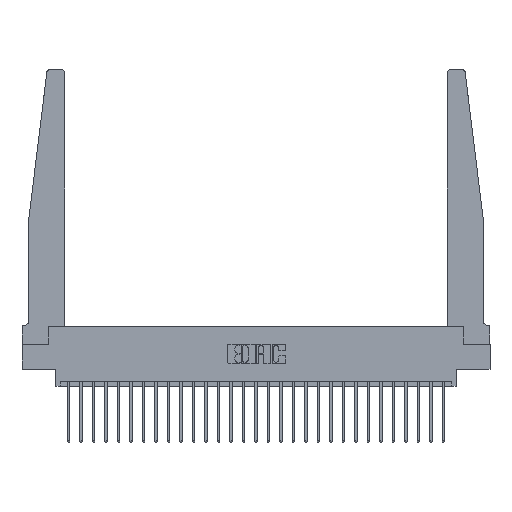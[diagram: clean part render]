
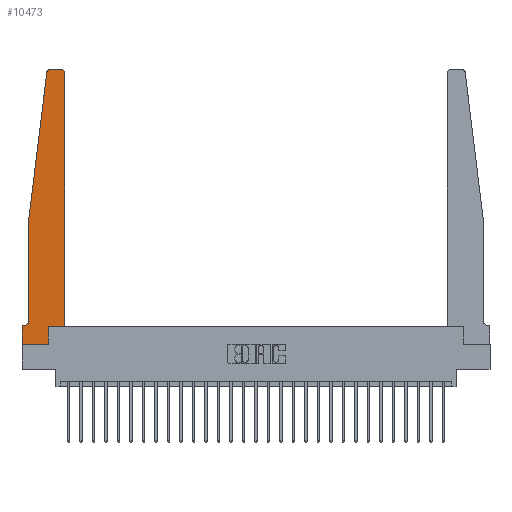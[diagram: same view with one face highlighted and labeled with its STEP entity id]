
A CAD part, top view. The second image highlights one B-rep face of the part: STEP entity #10473.
In plain terms, the highlighted planar face has unit normal (0, 0, 1).
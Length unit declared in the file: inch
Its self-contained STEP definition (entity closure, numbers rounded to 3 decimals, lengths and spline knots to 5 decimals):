
#105 = LINE ( 'NONE', #6262, #20757 ) ;
#352 = VERTEX_POINT ( 'NONE', #3799 ) ;
#757 = CARTESIAN_POINT ( 'NONE',  ( 0.065, 1.25, 0.37 ) ) ;
#1138 = CARTESIAN_POINT ( 'NONE',  ( 0.395, 2.72, 0.37 ) ) ;
#1237 = DIRECTION ( 'NONE',  ( 1., 0., 0. ) ) ;
#1488 = ORIENTED_EDGE ( 'NONE', *, *, #17526, .T. ) ;
#1494 = ORIENTED_EDGE ( 'NONE', *, *, #16974, .T. ) ;
#1615 = CARTESIAN_POINT ( 'NONE',  ( 0.425, 0.18, 0.37 ) ) ;
#2201 = VECTOR ( 'NONE', #18265, 39.37008 ) ;
#2873 = LINE ( 'NONE', #10935, #26638 ) ;
#2919 = ORIENTED_EDGE ( 'NONE', *, *, #4699, .T. ) ;
#3592 = DIRECTION ( 'NONE',  ( 0., 0., 1. ) ) ;
#3613 = CIRCLE ( 'NONE', #23729, 0.03 ) ;
#3799 = CARTESIAN_POINT ( 'NONE',  ( 0.27653, 2.75, 0.37 ) ) ;
#4699 = EDGE_CURVE ( 'NONE', #25485, #17885, #25501, .T. ) ;
#5096 = LINE ( 'NONE', #9466, #15453 ) ;
#5494 = EDGE_CURVE ( 'NONE', #25821, #16627, #105, .T. ) ;
#6005 = VERTEX_POINT ( 'NONE', #8654 ) ;
#6227 = EDGE_CURVE ( 'NONE', #9576, #12575, #3613, .T. ) ;
#6262 = CARTESIAN_POINT ( 'NONE',  ( 0.065, 1.25, 0.37 ) ) ;
#6812 = ORIENTED_EDGE ( 'NONE', *, *, #6227, .T. ) ;
#7024 = VECTOR ( 'NONE', #26680, 39.37008 ) ;
#7079 = EDGE_CURVE ( 'NONE', #22686, #25821, #5096, .T. ) ;
#7108 = CARTESIAN_POINT ( 'NONE',  ( 0., 0., 0.37 ) ) ;
#7135 = CARTESIAN_POINT ( 'NONE',  ( 0.425, 0.18, 0.37 ) ) ;
#7445 = DIRECTION ( 'NONE',  ( -1., 0., 0. ) ) ;
#7913 = DIRECTION ( 'NONE',  ( 0., -1., 0. ) ) ;
#8013 = CARTESIAN_POINT ( 'NONE',  ( 0.2605, 0., 0.37 ) ) ;
#8654 = CARTESIAN_POINT ( 'NONE',  ( 0., 0., 0.37 ) ) ;
#8744 = CARTESIAN_POINT ( 'NONE',  ( 0.24675, 2.72367, 0.37 ) ) ;
#9374 = ORIENTED_EDGE ( 'NONE', *, *, #5494, .T. ) ;
#9390 = CIRCLE ( 'NONE', #17277, 0.05 ) ;
#9466 = CARTESIAN_POINT ( 'NONE',  ( 0.065, 1.25, 0.37 ) ) ;
#9576 = VERTEX_POINT ( 'NONE', #15821 ) ;
#9884 = CARTESIAN_POINT ( 'NONE',  ( 0., 0., 0.37 ) ) ;
#10202 = VERTEX_POINT ( 'NONE', #23165 ) ;
#10473 = ADVANCED_FACE ( 'NONE', ( #23562 ), #24241, .T. ) ;
#10711 = EDGE_CURVE ( 'NONE', #6005, #17638, #11946, .T. ) ;
#10935 = CARTESIAN_POINT ( 'NONE',  ( 0.2605, 0.18, 0.37 ) ) ;
#11298 = ORIENTED_EDGE ( 'NONE', *, *, #25918, .T. ) ;
#11534 = DIRECTION ( 'NONE',  ( 1., 0., 0. ) ) ;
#11568 = LINE ( 'NONE', #11698, #14155 ) ;
#11698 = CARTESIAN_POINT ( 'NONE',  ( 0.065, 0.1875, 0.37 ) ) ;
#11766 = AXIS2_PLACEMENT_3D ( 'NONE', #22343, #18239, #20282 ) ;
#11946 = LINE ( 'NONE', #9884, #2201 ) ;
#12575 = VERTEX_POINT ( 'NONE', #14511 ) ;
#12731 = CARTESIAN_POINT ( 'NONE',  ( 0.2605, 0.18, 0.37 ) ) ;
#13665 = CARTESIAN_POINT ( 'NONE',  ( 0.015, 0.1875, 0.37 ) ) ;
#13770 = VECTOR ( 'NONE', #25782, 39.37008 ) ;
#13800 = EDGE_CURVE ( 'NONE', #16627, #20549, #9390, .T. ) ;
#14101 = VECTOR ( 'NONE', #23703, 39.37008 ) ;
#14127 = CARTESIAN_POINT ( 'NONE',  ( 0.425, 0.18, 0.37 ) ) ;
#14155 = VECTOR ( 'NONE', #7445, 39.37008 ) ;
#14511 = CARTESIAN_POINT ( 'NONE',  ( 0.395, 2.75, 0.37 ) ) ;
#15185 = ORIENTED_EDGE ( 'NONE', *, *, #23806, .T. ) ;
#15453 = VECTOR ( 'NONE', #15777, 39.37008 ) ;
#15749 = CARTESIAN_POINT ( 'NONE',  ( 0., 0.1875, 0.37 ) ) ;
#15777 = DIRECTION ( 'NONE',  ( -0.122, -0.992, 0. ) ) ;
#15821 = CARTESIAN_POINT ( 'NONE',  ( 0.425, 2.72, 0.37 ) ) ;
#16141 = ORIENTED_EDGE ( 'NONE', *, *, #23557, .T. ) ;
#16627 = VERTEX_POINT ( 'NONE', #21417 ) ;
#16889 = ORIENTED_EDGE ( 'NONE', *, *, #10711, .T. ) ;
#16974 = EDGE_CURVE ( 'NONE', #10202, #6005, #25893, .T. ) ;
#17246 = DIRECTION ( 'NONE',  ( 0., 1., 0. ) ) ;
#17277 = AXIS2_PLACEMENT_3D ( 'NONE', #21159, #25810, #19240 ) ;
#17526 = EDGE_CURVE ( 'NONE', #17885, #9576, #22290, .T. ) ;
#17602 = ORIENTED_EDGE ( 'NONE', *, *, #7079, .T. ) ;
#17638 = VERTEX_POINT ( 'NONE', #8013 ) ;
#17885 = VERTEX_POINT ( 'NONE', #14127 ) ;
#18018 = ORIENTED_EDGE ( 'NONE', *, *, #13800, .T. ) ;
#18239 = DIRECTION ( 'NONE',  ( 0., 0., 1. ) ) ;
#18256 = VECTOR ( 'NONE', #19832, 39.37008 ) ;
#18265 = DIRECTION ( 'NONE',  ( 1., 0., 0. ) ) ;
#18326 = CARTESIAN_POINT ( 'NONE',  ( 0.25, 2.75, 0.37 ) ) ;
#18826 = AXIS2_PLACEMENT_3D ( 'NONE', #15749, #20005, #1237 ) ;
#19240 = DIRECTION ( 'NONE',  ( -1., 0., 0. ) ) ;
#19832 = DIRECTION ( 'NONE',  ( 0., 1., 0. ) ) ;
#20005 = DIRECTION ( 'NONE',  ( 0., 0., 1. ) ) ;
#20282 = DIRECTION ( 'NONE',  ( 1., 0., 0. ) ) ;
#20519 = EDGE_CURVE ( 'NONE', #12575, #352, #26277, .T. ) ;
#20549 = VERTEX_POINT ( 'NONE', #13665 ) ;
#20757 = VECTOR ( 'NONE', #7913, 39.37008 ) ;
#21159 = CARTESIAN_POINT ( 'NONE',  ( 0.015, 0.2375, 0.37 ) ) ;
#21417 = CARTESIAN_POINT ( 'NONE',  ( 0.065, 0.2375, 0.37 ) ) ;
#21425 = ORIENTED_EDGE ( 'NONE', *, *, #20519, .T. ) ;
#22290 = LINE ( 'NONE', #1615, #18256 ) ;
#22343 = CARTESIAN_POINT ( 'NONE',  ( 0.27653, 2.72, 0.37 ) ) ;
#22686 = VERTEX_POINT ( 'NONE', #8744 ) ;
#23165 = CARTESIAN_POINT ( 'NONE',  ( 0., 0.1875, 0.37 ) ) ;
#23557 = EDGE_CURVE ( 'NONE', #352, #22686, #25312, .T. ) ;
#23562 = FACE_OUTER_BOUND ( 'NONE', #24168, .T. ) ;
#23703 = DIRECTION ( 'NONE',  ( 0., -1., 0. ) ) ;
#23729 = AXIS2_PLACEMENT_3D ( 'NONE', #1138, #3592, #11534 ) ;
#23806 = EDGE_CURVE ( 'NONE', #17638, #25485, #2873, .T. ) ;
#24168 = EDGE_LOOP ( 'NONE', ( #21425, #16141, #17602, #9374, #18018, #11298, #1494, #16889, #15185, #2919, #1488, #6812 ) ) ;
#24241 = PLANE ( 'NONE',  #18826 ) ;
#25312 = CIRCLE ( 'NONE', #11766, 0.03 ) ;
#25485 = VERTEX_POINT ( 'NONE', #12731 ) ;
#25501 = LINE ( 'NONE', #7135, #13770 ) ;
#25782 = DIRECTION ( 'NONE',  ( 1., 0., 0. ) ) ;
#25810 = DIRECTION ( 'NONE',  ( 0., 0., -1. ) ) ;
#25821 = VERTEX_POINT ( 'NONE', #757 ) ;
#25893 = LINE ( 'NONE', #7108, #14101 ) ;
#25918 = EDGE_CURVE ( 'NONE', #20549, #10202, #11568, .T. ) ;
#26277 = LINE ( 'NONE', #18326, #7024 ) ;
#26638 = VECTOR ( 'NONE', #17246, 39.37008 ) ;
#26680 = DIRECTION ( 'NONE',  ( -1., 0., 0. ) ) ;
